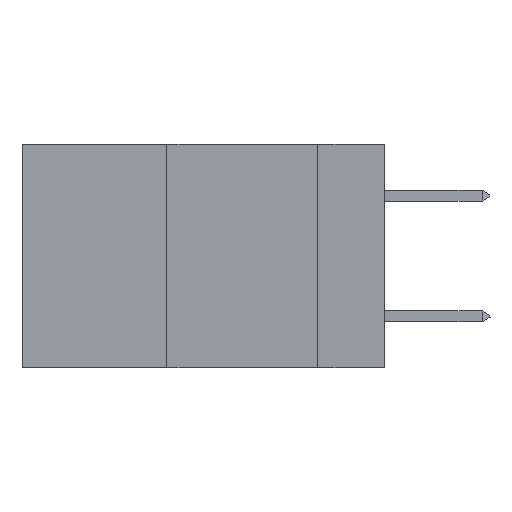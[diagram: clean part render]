
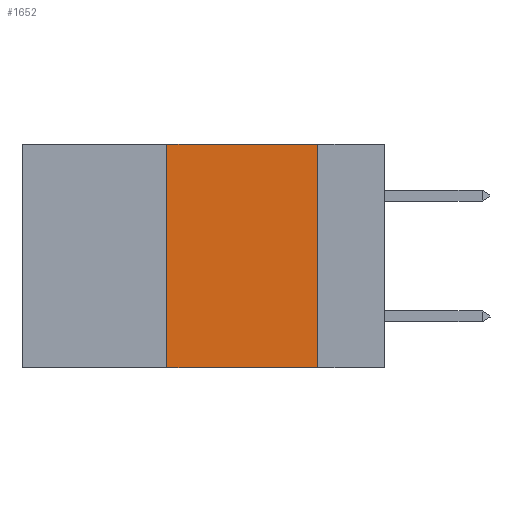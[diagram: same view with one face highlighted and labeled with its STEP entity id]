
A CAD part, left-side view. The second image highlights one B-rep face of the part: STEP entity #1652.
In plain terms, the highlighted planar face has unit normal (-1, 0, 0).
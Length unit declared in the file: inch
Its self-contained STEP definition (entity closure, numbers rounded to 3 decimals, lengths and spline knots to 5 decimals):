
#273 = CARTESIAN_POINT ( 'NONE',  ( 0., 0.36, 0. ) ) ;
#432 = VECTOR ( 'NONE', #2775, 39.37008 ) ;
#603 = FACE_OUTER_BOUND ( 'NONE', #3194, .T. ) ;
#1652 = ADVANCED_FACE ( 'NONE', ( #603 ), #8237, .F. ) ;
#2384 = DIRECTION ( 'NONE',  ( 0., 0., -1. ) ) ;
#2775 = DIRECTION ( 'NONE',  ( 0., -1., 0. ) ) ;
#3194 = EDGE_LOOP ( 'NONE', ( #13310, #17490, #10952, #4708 ) ) ;
#3441 = DIRECTION ( 'NONE',  ( 1., 0., 0. ) ) ;
#3468 = EDGE_CURVE ( 'NONE', #5948, #16111, #14700, .T. ) ;
#4708 = ORIENTED_EDGE ( 'NONE', *, *, #9175, .T. ) ;
#5571 = CARTESIAN_POINT ( 'NONE',  ( 0., 0.6, 0. ) ) ;
#5788 = CARTESIAN_POINT ( 'NONE',  ( 0., 0.11, 0. ) ) ;
#5948 = VERTEX_POINT ( 'NONE', #12887 ) ;
#7288 = DIRECTION ( 'NONE',  ( 0., 0., -1. ) ) ;
#7944 = CARTESIAN_POINT ( 'NONE',  ( 0., 0.11, 0. ) ) ;
#7979 = CARTESIAN_POINT ( 'NONE',  ( 0., 0.36, 0. ) ) ;
#8042 = DIRECTION ( 'NONE',  ( 0., 0., 1. ) ) ;
#8078 = VECTOR ( 'NONE', #17830, 39.37008 ) ;
#8237 = PLANE ( 'NONE',  #15162 ) ;
#8503 = VERTEX_POINT ( 'NONE', #5788 ) ;
#9175 = EDGE_CURVE ( 'NONE', #5948, #15402, #11837, .T. ) ;
#10395 = EDGE_CURVE ( 'NONE', #8503, #15402, #11156, .T. ) ;
#10625 = EDGE_CURVE ( 'NONE', #16111, #8503, #11371, .T. ) ;
#10952 = ORIENTED_EDGE ( 'NONE', *, *, #3468, .F. ) ;
#11059 = VECTOR ( 'NONE', #8042, 39.37008 ) ;
#11156 = LINE ( 'NONE', #7944, #17975 ) ;
#11371 = LINE ( 'NONE', #5571, #432 ) ;
#11837 = LINE ( 'NONE', #15095, #8078 ) ;
#12887 = CARTESIAN_POINT ( 'NONE',  ( 0., 0.36, -0.37 ) ) ;
#13310 = ORIENTED_EDGE ( 'NONE', *, *, #10395, .F. ) ;
#14325 = CARTESIAN_POINT ( 'NONE',  ( 0., 0.11, -0.37 ) ) ;
#14700 = LINE ( 'NONE', #7979, #11059 ) ;
#15095 = CARTESIAN_POINT ( 'NONE',  ( 0., 0.6, -0.37 ) ) ;
#15162 = AXIS2_PLACEMENT_3D ( 'NONE', #16929, #3441, #7288 ) ;
#15402 = VERTEX_POINT ( 'NONE', #14325 ) ;
#16111 = VERTEX_POINT ( 'NONE', #273 ) ;
#16929 = CARTESIAN_POINT ( 'NONE',  ( 0., 0.6, 0. ) ) ;
#17490 = ORIENTED_EDGE ( 'NONE', *, *, #10625, .F. ) ;
#17830 = DIRECTION ( 'NONE',  ( 0., -1., 0. ) ) ;
#17975 = VECTOR ( 'NONE', #2384, 39.37008 ) ;
